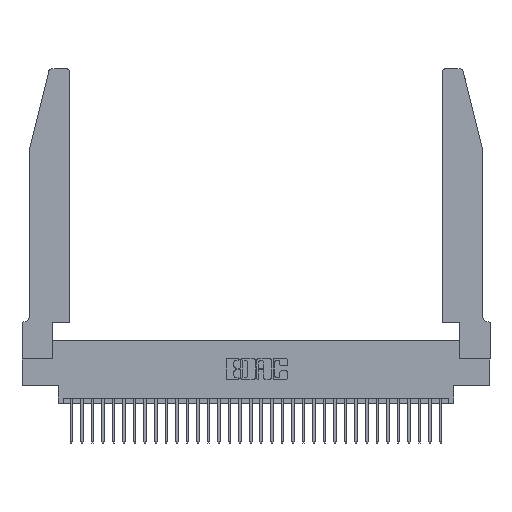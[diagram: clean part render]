
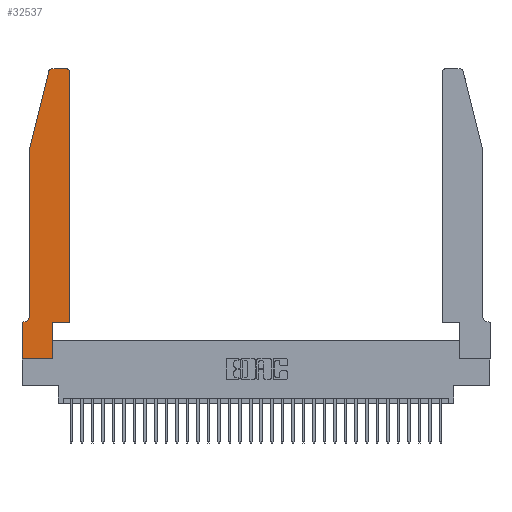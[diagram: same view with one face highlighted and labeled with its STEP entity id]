
A CAD part, top view. The second image highlights one B-rep face of the part: STEP entity #32537.
In plain terms, the highlighted planar face has unit normal (0, 0, 1).
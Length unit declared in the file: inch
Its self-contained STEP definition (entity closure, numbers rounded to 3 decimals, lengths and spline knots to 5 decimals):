
#574 = DIRECTION ( 'NONE',  ( -1., 0., 0. ) ) ;
#984 = CARTESIAN_POINT ( 'NONE',  ( 0.0755, 2., 0.37 ) ) ;
#1111 = DIRECTION ( 'NONE',  ( -0.239, -0.971, 0. ) ) ;
#1337 = VECTOR ( 'NONE', #1111, 39.37008 ) ;
#1716 = DIRECTION ( 'NONE',  ( -1., 0., 0. ) ) ;
#1760 = CARTESIAN_POINT ( 'NONE',  ( 0.0055, 0.42, 0.37 ) ) ;
#2236 = CARTESIAN_POINT ( 'NONE',  ( 0., 0.35, 0.37 ) ) ;
#2463 = FACE_OUTER_BOUND ( 'NONE', #20519, .T. ) ;
#2550 = AXIS2_PLACEMENT_3D ( 'NONE', #19356, #3621, #22005 ) ;
#2951 = DIRECTION ( 'NONE',  ( 0., -1., 0. ) ) ;
#3410 = CARTESIAN_POINT ( 'NONE',  ( 0.4505, 0.35, 0.37 ) ) ;
#3513 = ORIENTED_EDGE ( 'NONE', *, *, #6745, .T. ) ;
#3621 = DIRECTION ( 'NONE',  ( 0., 0., 1. ) ) ;
#3991 = VECTOR ( 'NONE', #32960, 39.37008 ) ;
#4437 = DIRECTION ( 'NONE',  ( -1., 0., 0. ) ) ;
#4457 = DIRECTION ( 'NONE',  ( 0., -1., 0. ) ) ;
#4694 = CARTESIAN_POINT ( 'NONE',  ( 0.284, 2.75, 0.37 ) ) ;
#5547 = LINE ( 'NONE', #5780, #24824 ) ;
#5780 = CARTESIAN_POINT ( 'NONE',  ( 0.4505, 0.35, 0.37 ) ) ;
#5937 = DIRECTION ( 'NONE',  ( 0., 0., 1. ) ) ;
#6120 = CARTESIAN_POINT ( 'NONE',  ( 0.0055, 0.35, 0.37 ) ) ;
#6745 = EDGE_CURVE ( 'NONE', #33548, #10791, #11195, .T. ) ;
#7415 = EDGE_CURVE ( 'NONE', #19346, #10128, #10746, .T. ) ;
#7468 = CARTESIAN_POINT ( 'NONE',  ( 0.4505, 0.35, 0.37 ) ) ;
#7485 = VERTEX_POINT ( 'NONE', #4694 ) ;
#8100 = CIRCLE ( 'NONE', #20713, 0.03 ) ;
#8374 = LINE ( 'NONE', #8963, #1337 ) ;
#8796 = DIRECTION ( 'NONE',  ( 0., 0., 1. ) ) ;
#8810 = VECTOR ( 'NONE', #2951, 39.37008 ) ;
#8963 = CARTESIAN_POINT ( 'NONE',  ( 0.0755, 2., 0.37 ) ) ;
#10128 = VERTEX_POINT ( 'NONE', #31066 ) ;
#10522 = EDGE_CURVE ( 'NONE', #23870, #20044, #8374, .T. ) ;
#10746 = LINE ( 'NONE', #17452, #16901 ) ;
#10791 = VERTEX_POINT ( 'NONE', #2236 ) ;
#10842 = ORIENTED_EDGE ( 'NONE', *, *, #10522, .T. ) ;
#11007 = ORIENTED_EDGE ( 'NONE', *, *, #22315, .T. ) ;
#11195 = LINE ( 'NONE', #22778, #30466 ) ;
#12368 = CARTESIAN_POINT ( 'NONE',  ( 0.25487, 2.72718, 0.37 ) ) ;
#12998 = CARTESIAN_POINT ( 'NONE',  ( 0.4505, 2.72, 0.37 ) ) ;
#14472 = EDGE_CURVE ( 'NONE', #19341, #19346, #23293, .T. ) ;
#14676 = CARTESIAN_POINT ( 'NONE',  ( 0., 0., 0.37 ) ) ;
#15046 = EDGE_CURVE ( 'NONE', #27204, #33548, #33828, .T. ) ;
#16050 = EDGE_CURVE ( 'NONE', #10128, #19695, #27866, .T. ) ;
#16219 = DIRECTION ( 'NONE',  ( 0., 1., 0. ) ) ;
#16351 = CARTESIAN_POINT ( 'NONE',  ( 0.2605, 2.75, 0.37 ) ) ;
#16578 = PLANE ( 'NONE',  #28472 ) ;
#16901 = VECTOR ( 'NONE', #25345, 39.37008 ) ;
#17182 = ORIENTED_EDGE ( 'NONE', *, *, #28816, .T. ) ;
#17452 = CARTESIAN_POINT ( 'NONE',  ( 0.2865, 0.35, 0.37 ) ) ;
#18272 = ORIENTED_EDGE ( 'NONE', *, *, #14472, .T. ) ;
#18406 = EDGE_CURVE ( 'NONE', #20044, #27204, #31821, .T. ) ;
#18519 = ORIENTED_EDGE ( 'NONE', *, *, #16050, .T. ) ;
#18762 = VECTOR ( 'NONE', #4457, 39.37008 ) ;
#18983 = CARTESIAN_POINT ( 'NONE',  ( 0., 0., 0.37 ) ) ;
#19236 = CARTESIAN_POINT ( 'NONE',  ( 0., 0.35, 0.37 ) ) ;
#19325 = EDGE_CURVE ( 'NONE', #19695, #31180, #5547, .T. ) ;
#19341 = VERTEX_POINT ( 'NONE', #18983 ) ;
#19346 = VERTEX_POINT ( 'NONE', #21970 ) ;
#19356 = CARTESIAN_POINT ( 'NONE',  ( 0.4205, 2.72, 0.37 ) ) ;
#19695 = VERTEX_POINT ( 'NONE', #7468 ) ;
#20044 = VERTEX_POINT ( 'NONE', #984 ) ;
#20174 = DIRECTION ( 'NONE',  ( 0., 0., -1. ) ) ;
#20260 = ORIENTED_EDGE ( 'NONE', *, *, #33008, .T. ) ;
#20465 = VERTEX_POINT ( 'NONE', #25991 ) ;
#20519 = EDGE_LOOP ( 'NONE', ( #11007, #17182, #10842, #27599, #33930, #3513, #23615, #18272, #27062, #18519, #22893, #20260 ) ) ;
#20713 = AXIS2_PLACEMENT_3D ( 'NONE', #21675, #5937, #24279 ) ;
#21348 = CARTESIAN_POINT ( 'NONE',  ( 0., 0., 0.37 ) ) ;
#21675 = CARTESIAN_POINT ( 'NONE',  ( 0.284, 2.72, 0.37 ) ) ;
#21970 = CARTESIAN_POINT ( 'NONE',  ( 0.2865, 0., 0.37 ) ) ;
#22005 = DIRECTION ( 'NONE',  ( 1., 0., 0. ) ) ;
#22293 = LINE ( 'NONE', #16351, #23095 ) ;
#22315 = EDGE_CURVE ( 'NONE', #20465, #7485, #22293, .T. ) ;
#22778 = CARTESIAN_POINT ( 'NONE',  ( 0.0755, 0.35, 0.37 ) ) ;
#22893 = ORIENTED_EDGE ( 'NONE', *, *, #19325, .T. ) ;
#23095 = VECTOR ( 'NONE', #574, 39.37008 ) ;
#23293 = LINE ( 'NONE', #14676, #3991 ) ;
#23615 = ORIENTED_EDGE ( 'NONE', *, *, #26804, .T. ) ;
#23870 = VERTEX_POINT ( 'NONE', #12368 ) ;
#24279 = DIRECTION ( 'NONE',  ( 1., 0., 0. ) ) ;
#24824 = VECTOR ( 'NONE', #16219, 39.37008 ) ;
#25251 = AXIS2_PLACEMENT_3D ( 'NONE', #1760, #20174, #4437 ) ;
#25345 = DIRECTION ( 'NONE',  ( 0., 1., 0. ) ) ;
#25437 = CARTESIAN_POINT ( 'NONE',  ( 0.0755, 2., 0.37 ) ) ;
#25991 = CARTESIAN_POINT ( 'NONE',  ( 0.4205, 2.75, 0.37 ) ) ;
#26804 = EDGE_CURVE ( 'NONE', #10791, #19341, #29701, .T. ) ;
#27049 = VECTOR ( 'NONE', #32143, 39.37008 ) ;
#27062 = ORIENTED_EDGE ( 'NONE', *, *, #7415, .T. ) ;
#27121 = DIRECTION ( 'NONE',  ( 1., 0., 0. ) ) ;
#27204 = VERTEX_POINT ( 'NONE', #28267 ) ;
#27599 = ORIENTED_EDGE ( 'NONE', *, *, #18406, .T. ) ;
#27866 = LINE ( 'NONE', #3410, #27049 ) ;
#28267 = CARTESIAN_POINT ( 'NONE',  ( 0.0755, 0.42, 0.37 ) ) ;
#28472 = AXIS2_PLACEMENT_3D ( 'NONE', #19236, #8796, #27121 ) ;
#28816 = EDGE_CURVE ( 'NONE', #7485, #23870, #8100, .T. ) ;
#29154 = CIRCLE ( 'NONE', #2550, 0.03 ) ;
#29701 = LINE ( 'NONE', #21348, #8810 ) ;
#30466 = VECTOR ( 'NONE', #1716, 39.37008 ) ;
#31066 = CARTESIAN_POINT ( 'NONE',  ( 0.2865, 0.35, 0.37 ) ) ;
#31180 = VERTEX_POINT ( 'NONE', #12998 ) ;
#31821 = LINE ( 'NONE', #25437, #18762 ) ;
#32143 = DIRECTION ( 'NONE',  ( 1., 0., 0. ) ) ;
#32537 = ADVANCED_FACE ( 'NONE', ( #2463 ), #16578, .T. ) ;
#32960 = DIRECTION ( 'NONE',  ( 1., 0., 0. ) ) ;
#33008 = EDGE_CURVE ( 'NONE', #31180, #20465, #29154, .T. ) ;
#33548 = VERTEX_POINT ( 'NONE', #6120 ) ;
#33828 = CIRCLE ( 'NONE', #25251, 0.07 ) ;
#33930 = ORIENTED_EDGE ( 'NONE', *, *, #15046, .T. ) ;
